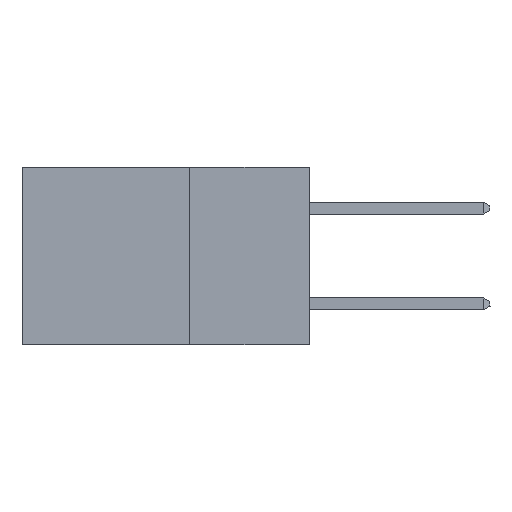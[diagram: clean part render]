
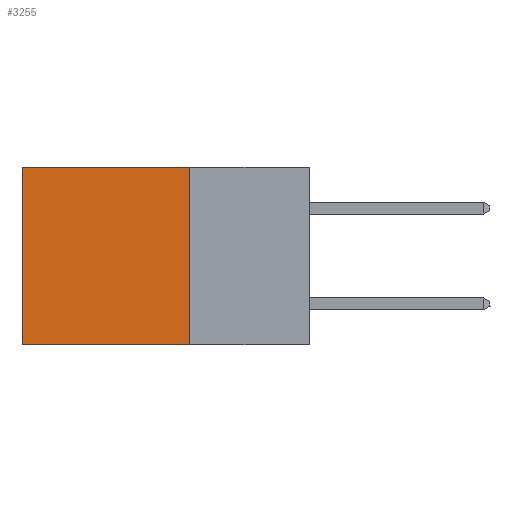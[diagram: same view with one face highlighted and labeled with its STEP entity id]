
A CAD part, left-side view. The second image highlights one B-rep face of the part: STEP entity #3255.
In plain terms, the highlighted planar face has unit normal (-1, 0, 0).
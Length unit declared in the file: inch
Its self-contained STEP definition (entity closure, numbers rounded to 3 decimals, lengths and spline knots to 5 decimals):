
#566 = CARTESIAN_POINT ( 'NONE',  ( 0.2875, 0.6, -0.37 ) ) ;
#3255 = ADVANCED_FACE ( 'NONE', ( #11867 ), #16799, .F. ) ;
#4202 = VECTOR ( 'NONE', #25686, 39.37008 ) ;
#4811 = ORIENTED_EDGE ( 'NONE', *, *, #33073, .F. ) ;
#5584 = DIRECTION ( 'NONE',  ( 0., 1., 0. ) ) ;
#5688 = VERTEX_POINT ( 'NONE', #26773 ) ;
#5706 = LINE ( 'NONE', #15535, #31493 ) ;
#6399 = EDGE_CURVE ( 'NONE', #31263, #5688, #7594, .T. ) ;
#7433 = LINE ( 'NONE', #20304, #27443 ) ;
#7594 = LINE ( 'NONE', #17593, #4202 ) ;
#9338 = CARTESIAN_POINT ( 'NONE',  ( 0.2875, 0.25, 0. ) ) ;
#10447 = DIRECTION ( 'NONE',  ( 0., 0., -1. ) ) ;
#11194 = CARTESIAN_POINT ( 'NONE',  ( 0.2875, 0.6, 0. ) ) ;
#11867 = FACE_OUTER_BOUND ( 'NONE', #23977, .T. ) ;
#11971 = VERTEX_POINT ( 'NONE', #566 ) ;
#14335 = AXIS2_PLACEMENT_3D ( 'NONE', #9338, #24396, #26772 ) ;
#15082 = CARTESIAN_POINT ( 'NONE',  ( 0.2875, 0.25, 0. ) ) ;
#15367 = EDGE_CURVE ( 'NONE', #31025, #11971, #5706, .T. ) ;
#15535 = CARTESIAN_POINT ( 'NONE',  ( 0.2875, 0.6, 0. ) ) ;
#16799 = PLANE ( 'NONE',  #14335 ) ;
#17593 = CARTESIAN_POINT ( 'NONE',  ( 0.2875, 0.25, 0. ) ) ;
#18799 = CARTESIAN_POINT ( 'NONE',  ( 0.2875, 0.25, 0. ) ) ;
#20304 = CARTESIAN_POINT ( 'NONE',  ( 0.2875, 0.25, -0.37 ) ) ;
#23977 = EDGE_LOOP ( 'NONE', ( #24723, #4811, #31030, #24476 ) ) ;
#24396 = DIRECTION ( 'NONE',  ( 1., 0., 0. ) ) ;
#24476 = ORIENTED_EDGE ( 'NONE', *, *, #26093, .T. ) ;
#24723 = ORIENTED_EDGE ( 'NONE', *, *, #15367, .T. ) ;
#25686 = DIRECTION ( 'NONE',  ( 0., 0., -1. ) ) ;
#26093 = EDGE_CURVE ( 'NONE', #31263, #31025, #28773, .T. ) ;
#26772 = DIRECTION ( 'NONE',  ( 0., 0., -1. ) ) ;
#26773 = CARTESIAN_POINT ( 'NONE',  ( 0.2875, 0.25, -0.37 ) ) ;
#26880 = VECTOR ( 'NONE', #5584, 39.37008 ) ;
#27443 = VECTOR ( 'NONE', #31089, 39.37008 ) ;
#28773 = LINE ( 'NONE', #18799, #26880 ) ;
#31025 = VERTEX_POINT ( 'NONE', #11194 ) ;
#31030 = ORIENTED_EDGE ( 'NONE', *, *, #6399, .F. ) ;
#31089 = DIRECTION ( 'NONE',  ( 0., 1., 0. ) ) ;
#31263 = VERTEX_POINT ( 'NONE', #15082 ) ;
#31493 = VECTOR ( 'NONE', #10447, 39.37008 ) ;
#33073 = EDGE_CURVE ( 'NONE', #5688, #11971, #7433, .T. ) ;
